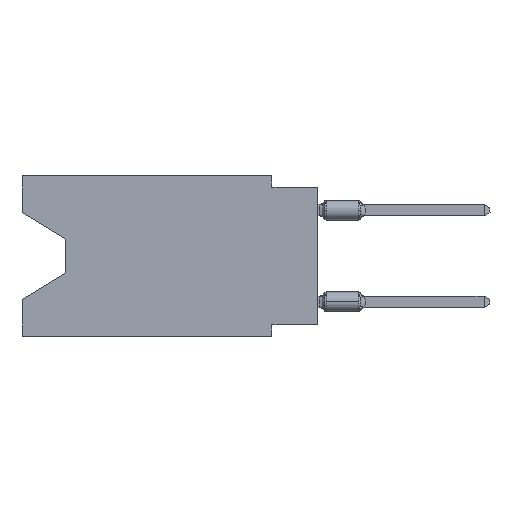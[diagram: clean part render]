
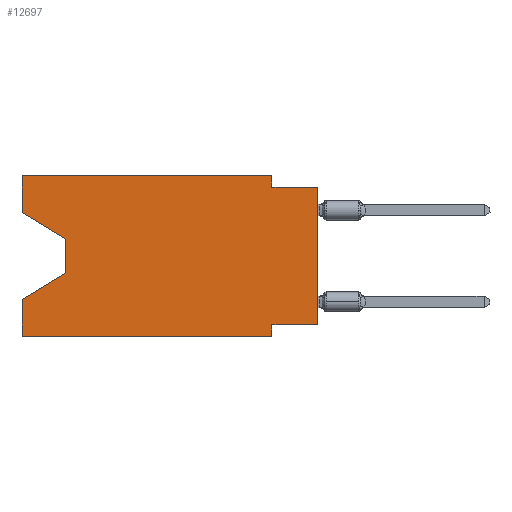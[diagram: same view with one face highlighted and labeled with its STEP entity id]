
A CAD part, left-side view. The second image highlights one B-rep face of the part: STEP entity #12697.
In plain terms, the highlighted planar face has unit normal (-1, 0, 0).
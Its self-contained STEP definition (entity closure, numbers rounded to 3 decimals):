
#163 = VERTEX_POINT ( 'NONE', #4088 ) ;
#312 = LINE ( 'NONE', #2221, #11352 ) ;
#497 = DIRECTION ( 'NONE',  ( 0., 0., 1. ) ) ;
#613 = DIRECTION ( 'NONE',  ( 0., -1., 0. ) ) ;
#667 = CARTESIAN_POINT ( 'NONE',  ( 0., 16.383, -2.038 ) ) ;
#677 = EDGE_LOOP ( 'NONE', ( #15993, #16162, #17370, #18065, #16701, #13436, #6507, #12537, #14642, #15462, #14170, #15707 ) ) ;
#1278 = DIRECTION ( 'NONE',  ( 0., 0., 1. ) ) ;
#1927 = DIRECTION ( 'NONE',  ( 0., 0., -1. ) ) ;
#2221 = CARTESIAN_POINT ( 'NONE',  ( 0., 16.383, -2.038 ) ) ;
#2326 = CARTESIAN_POINT ( 'NONE',  ( 0., 16.383, -8.89 ) ) ;
#2705 = AXIS2_PLACEMENT_3D ( 'NONE', #16311, #10262, #19216 ) ;
#2966 = LINE ( 'NONE', #12839, #4046 ) ;
#3286 = LINE ( 'NONE', #11241, #3779 ) ;
#3505 = DIRECTION ( 'NONE',  ( 0., -0.855, -0.519 ) ) ;
#3515 = CARTESIAN_POINT ( 'NONE',  ( 0., 2.54, 0. ) ) ;
#3765 = DIRECTION ( 'NONE',  ( 0., 0., -1. ) ) ;
#3779 = VECTOR ( 'NONE', #18601, 1000. ) ;
#4046 = VECTOR ( 'NONE', #13409, 1000. ) ;
#4088 = CARTESIAN_POINT ( 'NONE',  ( 0., 2.54, -8.255 ) ) ;
#4146 = DIRECTION ( 'NONE',  ( 0., 0.855, -0.519 ) ) ;
#4167 = VERTEX_POINT ( 'NONE', #12951 ) ;
#4321 = CARTESIAN_POINT ( 'NONE',  ( 0., 16.383, 0. ) ) ;
#4565 = DIRECTION ( 'NONE',  ( 0., -1., 0. ) ) ;
#4669 = LINE ( 'NONE', #18197, #8498 ) ;
#4672 = DIRECTION ( 'NONE',  ( 0., -1., 0. ) ) ;
#5142 = EDGE_CURVE ( 'NONE', #15815, #13885, #312, .T. ) ;
#5224 = EDGE_CURVE ( 'NONE', #15450, #6760, #18443, .T. ) ;
#5313 = EDGE_CURVE ( 'NONE', #163, #4167, #2966, .T. ) ;
#5563 = LINE ( 'NONE', #11637, #15742 ) ;
#5792 = CARTESIAN_POINT ( 'NONE',  ( 0., 13.97, -3.505 ) ) ;
#6374 = VERTEX_POINT ( 'NONE', #18446 ) ;
#6500 = EDGE_CURVE ( 'NONE', #17275, #9948, #9497, .T. ) ;
#6507 = ORIENTED_EDGE ( 'NONE', *, *, #6947, .F. ) ;
#6760 = VERTEX_POINT ( 'NONE', #8882 ) ;
#6870 = VECTOR ( 'NONE', #17265, 1000. ) ;
#6947 = EDGE_CURVE ( 'NONE', #18955, #163, #3286, .T. ) ;
#7177 = PLANE ( 'NONE',  #2705 ) ;
#8485 = CARTESIAN_POINT ( 'NONE',  ( 0., 2.54, -0.635 ) ) ;
#8498 = VECTOR ( 'NONE', #4565, 1000. ) ;
#8882 = CARTESIAN_POINT ( 'NONE',  ( 0., 16.383, -6.852 ) ) ;
#8965 = LINE ( 'NONE', #13516, #13178 ) ;
#9435 = LINE ( 'NONE', #12706, #6870 ) ;
#9497 = LINE ( 'NONE', #15732, #16461 ) ;
#9563 = CARTESIAN_POINT ( 'NONE',  ( 0., 0., -0.635 ) ) ;
#9852 = CARTESIAN_POINT ( 'NONE',  ( 0., 13.97, -3.505 ) ) ;
#9881 = CARTESIAN_POINT ( 'NONE',  ( 0., 2.54, 0. ) ) ;
#9948 = VERTEX_POINT ( 'NONE', #9881 ) ;
#10164 = VERTEX_POINT ( 'NONE', #9563 ) ;
#10262 = DIRECTION ( 'NONE',  ( 1., 0., 0. ) ) ;
#10665 = VECTOR ( 'NONE', #4146, 1000. ) ;
#11117 = VERTEX_POINT ( 'NONE', #8485 ) ;
#11241 = CARTESIAN_POINT ( 'NONE',  ( 0., 0., -8.255 ) ) ;
#11352 = VECTOR ( 'NONE', #3505, 1000. ) ;
#11440 = LINE ( 'NONE', #9852, #15138 ) ;
#11613 = CARTESIAN_POINT ( 'NONE',  ( 0., 13.97, -5.385 ) ) ;
#11637 = CARTESIAN_POINT ( 'NONE',  ( 0., 0., 0. ) ) ;
#12396 = EDGE_CURVE ( 'NONE', #9948, #11117, #15641, .T. ) ;
#12537 = ORIENTED_EDGE ( 'NONE', *, *, #13156, .T. ) ;
#12697 = ADVANCED_FACE ( 'NONE', ( #13133 ), #7177, .F. ) ;
#12706 = CARTESIAN_POINT ( 'NONE',  ( 0., 16.383, 0. ) ) ;
#12839 = CARTESIAN_POINT ( 'NONE',  ( 0., 2.54, -8.89 ) ) ;
#12951 = CARTESIAN_POINT ( 'NONE',  ( 0., 2.54, -8.89 ) ) ;
#13009 = LINE ( 'NONE', #11613, #10665 ) ;
#13133 = FACE_OUTER_BOUND ( 'NONE', #677, .T. ) ;
#13156 = EDGE_CURVE ( 'NONE', #18955, #10164, #5563, .T. ) ;
#13178 = VECTOR ( 'NONE', #4672, 1000. ) ;
#13409 = DIRECTION ( 'NONE',  ( 0., 0., -1. ) ) ;
#13436 = ORIENTED_EDGE ( 'NONE', *, *, #5313, .F. ) ;
#13491 = EDGE_CURVE ( 'NONE', #6374, #6760, #13009, .T. ) ;
#13516 = CARTESIAN_POINT ( 'NONE',  ( 0., 16.383, -8.89 ) ) ;
#13885 = VERTEX_POINT ( 'NONE', #5792 ) ;
#14170 = ORIENTED_EDGE ( 'NONE', *, *, #6500, .F. ) ;
#14204 = VECTOR ( 'NONE', #497, 1000. ) ;
#14504 = EDGE_CURVE ( 'NONE', #11117, #10164, #4669, .T. ) ;
#14582 = EDGE_CURVE ( 'NONE', #13885, #6374, #11440, .T. ) ;
#14642 = ORIENTED_EDGE ( 'NONE', *, *, #14504, .F. ) ;
#15138 = VECTOR ( 'NONE', #3765, 1000. ) ;
#15450 = VERTEX_POINT ( 'NONE', #2326 ) ;
#15462 = ORIENTED_EDGE ( 'NONE', *, *, #12396, .F. ) ;
#15641 = LINE ( 'NONE', #3515, #19214 ) ;
#15707 = ORIENTED_EDGE ( 'NONE', *, *, #18894, .F. ) ;
#15732 = CARTESIAN_POINT ( 'NONE',  ( 0., 16.383, 0. ) ) ;
#15742 = VECTOR ( 'NONE', #1278, 1000. ) ;
#15815 = VERTEX_POINT ( 'NONE', #667 ) ;
#15993 = ORIENTED_EDGE ( 'NONE', *, *, #5142, .T. ) ;
#16162 = ORIENTED_EDGE ( 'NONE', *, *, #14582, .T. ) ;
#16311 = CARTESIAN_POINT ( 'NONE',  ( 0., 16.383, 0. ) ) ;
#16461 = VECTOR ( 'NONE', #613, 1000. ) ;
#16701 = ORIENTED_EDGE ( 'NONE', *, *, #18219, .T. ) ;
#17218 = CARTESIAN_POINT ( 'NONE',  ( 0., 16.383, 0. ) ) ;
#17265 = DIRECTION ( 'NONE',  ( 0., 0., 1. ) ) ;
#17275 = VERTEX_POINT ( 'NONE', #4321 ) ;
#17370 = ORIENTED_EDGE ( 'NONE', *, *, #13491, .T. ) ;
#18065 = ORIENTED_EDGE ( 'NONE', *, *, #5224, .F. ) ;
#18197 = CARTESIAN_POINT ( 'NONE',  ( 0., 0., -0.635 ) ) ;
#18219 = EDGE_CURVE ( 'NONE', #15450, #4167, #8965, .T. ) ;
#18443 = LINE ( 'NONE', #17218, #14204 ) ;
#18446 = CARTESIAN_POINT ( 'NONE',  ( 0., 13.97, -5.385 ) ) ;
#18601 = DIRECTION ( 'NONE',  ( 0., 1., 0. ) ) ;
#18894 = EDGE_CURVE ( 'NONE', #15815, #17275, #9435, .T. ) ;
#18955 = VERTEX_POINT ( 'NONE', #19520 ) ;
#19214 = VECTOR ( 'NONE', #1927, 1000. ) ;
#19216 = DIRECTION ( 'NONE',  ( 0., 0., -1. ) ) ;
#19520 = CARTESIAN_POINT ( 'NONE',  ( 0., 0., -8.255 ) ) ;
